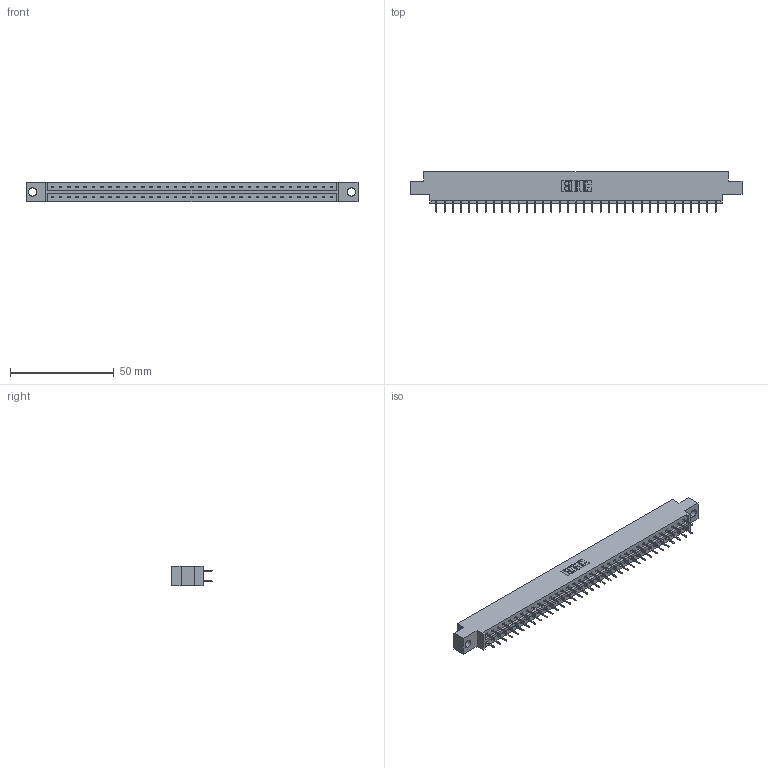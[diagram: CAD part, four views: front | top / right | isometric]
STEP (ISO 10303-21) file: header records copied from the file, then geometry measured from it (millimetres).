
FILE_DESCRIPTION (( 'STEP AP203' ), '1' );
FILE_NAME ('333-070-524-804.STEP', '2018-08-04T14:37:53', ( '' ), ( '' ), 'SwSTEP 2.0', 'SolidWorks 2016', '' );
FILE_SCHEMA (( 'CONFIG_CONTROL_DESIGN' ));
Length unit declared in the file: inch
Products named in the file (3): 333 Part_Offset - .156 Dia - TH; 345-292-001_345-293-124; 333-070-524-804
Assembly tree (71 placements, depth 2):
  333-070-524-804
    333 Part_Offset - .156 Dia - TH
    345-292-001_345-293-124  x70
Bounding box: 160.22 x 19.69 x 9.4 mm (x, y, z)
Volume: 15870.8 mm3; surface area: 18390.4 mm2
Topology: 71 solids, 71 shells, 4038 faces, 11453 edges, 7354 vertices
Faces by surface type: plane 3014, cylinder 1024
Entity records: 23631 total; most frequent: CARTESIAN_POINT 3926, ORIENTED_EDGE 3862, DIRECTION 3367, EDGE_CURVE 1931, VECTOR 1807, LINE 1807, VERTEX_POINT 1282, AXIS2_PLACEMENT_3D 780
